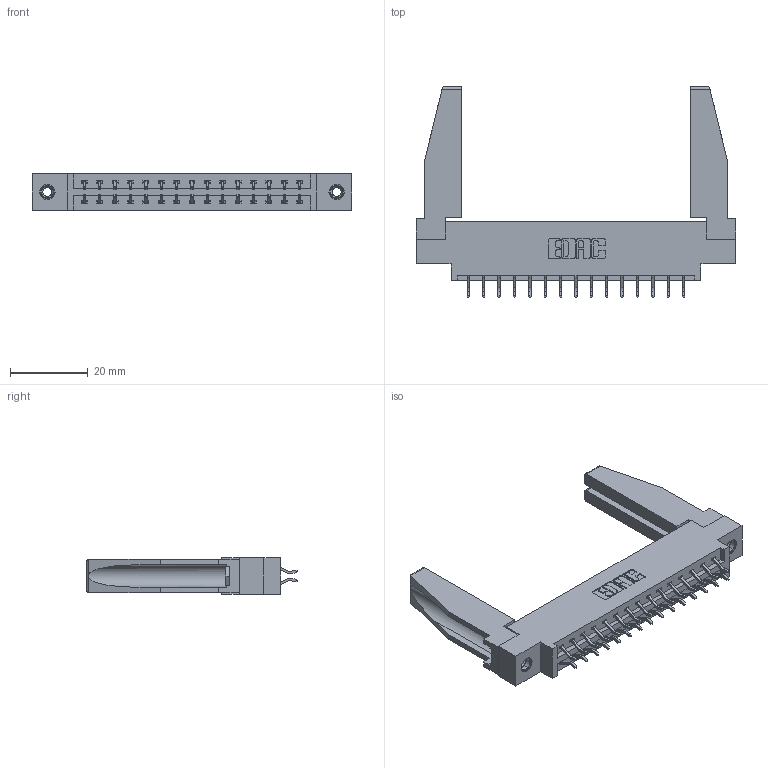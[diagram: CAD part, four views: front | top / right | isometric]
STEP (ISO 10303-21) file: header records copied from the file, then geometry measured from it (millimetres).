
FILE_DESCRIPTION (( 'STEP AP203' ), '1' );
FILE_NAME ('387-030-556-878.STEP', '2019-10-17T14:59:51', ( '' ), ( '' ), 'SwSTEP 2.0', 'SolidWorks 2016', '' );
FILE_SCHEMA (( 'CONFIG_CONTROL_DESIGN' ));
Length unit declared in the file: inch
Products named in the file (5): 345-292-001_556 Tail; 387-030-556-878; 337 Part_0.170 Offset - 0.156 Dia-TI; 307-220-078; 345-250-001_345-250-001-102
Assembly tree (35 placements, depth 2):
  387-030-556-878
    337 Part_0.170 Offset - 0.156 Dia-TI
    345-292-001_556 Tail  x30
    345-250-001_345-250-001-102  x2
    307-220-078  x2
Bounding box: 82.45 x 54.37 x 9.4 mm (x, y, z)
Volume: 12204.3 mm3; surface area: 12926.9 mm2
Topology: 35 solids, 35 shells, 2048 faces, 6023 edges, 3966 vertices
Faces by surface type: plane 1418, cylinder 614, cone 12, torus 4
Entity records: 17914 total; most frequent: CARTESIAN_POINT 3056, ORIENTED_EDGE 2936, DIRECTION 2644, EDGE_CURVE 1468, VECTOR 1294, LINE 1294, VERTEX_POINT 972, AXIS2_PLACEMENT_3D 675
